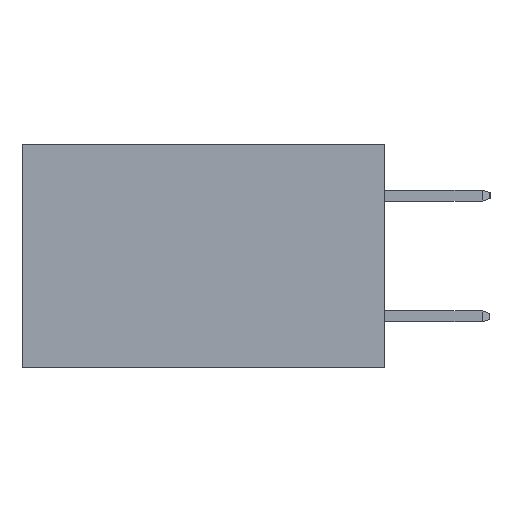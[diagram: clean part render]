
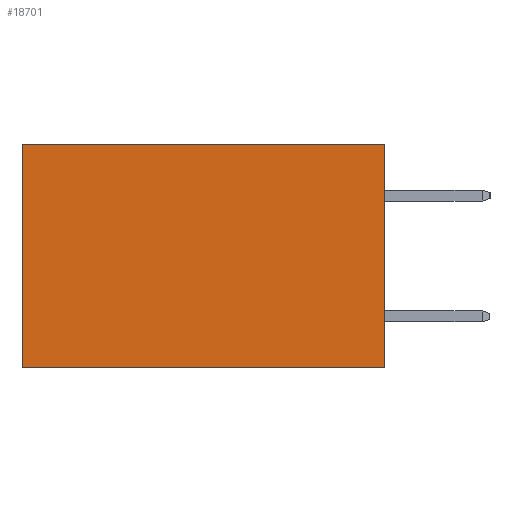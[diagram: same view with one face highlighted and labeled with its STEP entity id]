
A CAD part, left-side view. The second image highlights one B-rep face of the part: STEP entity #18701.
In plain terms, the highlighted planar face has unit normal (-1, 0, 0).
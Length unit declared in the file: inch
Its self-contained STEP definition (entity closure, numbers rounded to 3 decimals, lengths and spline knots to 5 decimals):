
#590 = VECTOR ( 'NONE', #4477, 39.37008 ) ;
#1466 = EDGE_CURVE ( 'NONE', #19804, #26298, #26040, .T. ) ;
#1562 = DIRECTION ( 'NONE',  ( 0., 1., 0. ) ) ;
#2057 = EDGE_CURVE ( 'NONE', #26298, #26882, #17120, .T. ) ;
#2478 = EDGE_LOOP ( 'NONE', ( #6523, #25776, #5415, #7414 ) ) ;
#2685 = FACE_OUTER_BOUND ( 'NONE', #2478, .T. ) ;
#3330 = VECTOR ( 'NONE', #5355, 39.37008 ) ;
#4115 = VERTEX_POINT ( 'NONE', #8880 ) ;
#4477 = DIRECTION ( 'NONE',  ( 0., 0., -1. ) ) ;
#5355 = DIRECTION ( 'NONE',  ( 0., 1., 0. ) ) ;
#5364 = VECTOR ( 'NONE', #22270, 39.37008 ) ;
#5415 = ORIENTED_EDGE ( 'NONE', *, *, #26920, .F. ) ;
#6053 = CARTESIAN_POINT ( 'NONE',  ( 0.298, 0., 0. ) ) ;
#6523 = ORIENTED_EDGE ( 'NONE', *, *, #2057, .T. ) ;
#7414 = ORIENTED_EDGE ( 'NONE', *, *, #1466, .T. ) ;
#8880 = CARTESIAN_POINT ( 'NONE',  ( 0.298, 0., -0.37 ) ) ;
#11678 = CARTESIAN_POINT ( 'NONE',  ( 0.298, 0., -0.37 ) ) ;
#11824 = LINE ( 'NONE', #23262, #590 ) ;
#12224 = DIRECTION ( 'NONE',  ( 1., 0., 0. ) ) ;
#14447 = LINE ( 'NONE', #11678, #3330 ) ;
#16180 = VECTOR ( 'NONE', #1562, 39.37008 ) ;
#16820 = CARTESIAN_POINT ( 'NONE',  ( 0.298, 0.6, -0.37 ) ) ;
#17120 = LINE ( 'NONE', #21858, #5364 ) ;
#18701 = ADVANCED_FACE ( 'NONE', ( #2685 ), #22681, .F. ) ;
#19086 = CARTESIAN_POINT ( 'NONE',  ( 0.298, 0., 0. ) ) ;
#19804 = VERTEX_POINT ( 'NONE', #6053 ) ;
#21158 = AXIS2_PLACEMENT_3D ( 'NONE', #24767, #12224, #26883 ) ;
#21858 = CARTESIAN_POINT ( 'NONE',  ( 0.298, 0.6, 0. ) ) ;
#22270 = DIRECTION ( 'NONE',  ( 0., 0., -1. ) ) ;
#22681 = PLANE ( 'NONE',  #21158 ) ;
#23105 = CARTESIAN_POINT ( 'NONE',  ( 0.298, 0.6, 0. ) ) ;
#23262 = CARTESIAN_POINT ( 'NONE',  ( 0.298, 0., 0. ) ) ;
#24767 = CARTESIAN_POINT ( 'NONE',  ( 0.298, 0., 0. ) ) ;
#25776 = ORIENTED_EDGE ( 'NONE', *, *, #25974, .F. ) ;
#25974 = EDGE_CURVE ( 'NONE', #4115, #26882, #14447, .T. ) ;
#26040 = LINE ( 'NONE', #19086, #16180 ) ;
#26298 = VERTEX_POINT ( 'NONE', #23105 ) ;
#26882 = VERTEX_POINT ( 'NONE', #16820 ) ;
#26883 = DIRECTION ( 'NONE',  ( 0., 0., -1. ) ) ;
#26920 = EDGE_CURVE ( 'NONE', #19804, #4115, #11824, .T. ) ;
